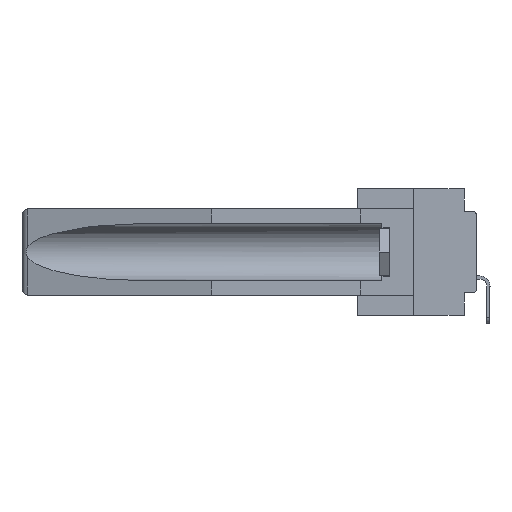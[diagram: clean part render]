
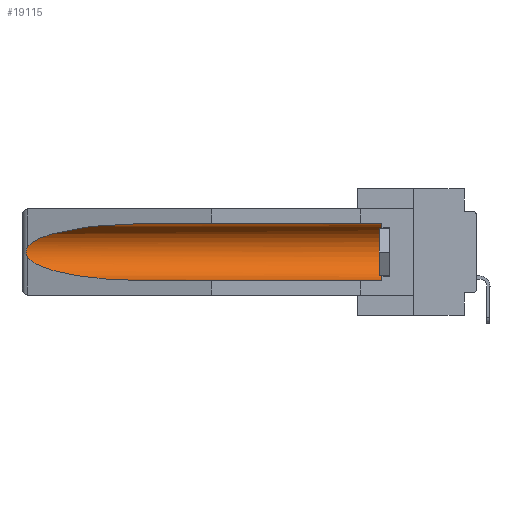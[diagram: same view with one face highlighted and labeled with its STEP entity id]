
A CAD part, left-side view. The second image highlights one B-rep face of the part: STEP entity #19115.
In plain terms, the highlighted cylindrical face has radius 2.857 mm (diameter 5.715 mm), a partial arc.
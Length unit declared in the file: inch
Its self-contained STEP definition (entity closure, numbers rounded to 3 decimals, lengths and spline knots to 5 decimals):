
#19 = ORIENTED_EDGE ( 'NONE', *, *, #5161, .T. ) ;
#198 = ORIENTED_EDGE ( 'NONE', *, *, #28148, .T. ) ;
#740 = CYLINDRICAL_SURFACE ( 'NONE', #19014, 0.1125 ) ;
#1130 = B_SPLINE_CURVE_WITH_KNOTS ( 'NONE', 3,
 ( #10382, #30782, #22417, #28241, #13743, #25695, #16826, #25834, #5448, #13874 ),
 .UNSPECIFIED., .F., .F.,
 ( 4, 2, 2, 2, 4 ),
 ( 0., 0.00029, 0.00058, 0.00087, 0.00117 ),
 .UNSPECIFIED. ) ;
#1385 = DIRECTION ( 'NONE',  ( 0., 1., 0. ) ) ;
#1723 =( BOUNDED_CURVE ( )  B_SPLINE_CURVE ( 3, ( #23127, #3036, #36189, #18755 ),
 .UNSPECIFIED., .F., .F. ) 
 B_SPLINE_CURVE_WITH_KNOTS ( ( 4, 4 ),
 ( 0.1948, 1.5708 ),
 .UNSPECIFIED. ) 
 CURVE ( )  GEOMETRIC_REPRESENTATION_ITEM ( )  RATIONAL_B_SPLINE_CURVE ( ( 1., 0.848, 0.848, 1. ) ) 
 REPRESENTATION_ITEM ( '' )  );
#3028 = ORIENTED_EDGE ( 'NONE', *, *, #11468, .T. ) ;
#3036 = CARTESIAN_POINT ( 'NONE',  ( 0.25451, 1.48313, -0.24835 ) ) ;
#4368 = CARTESIAN_POINT ( 'NONE',  ( 0.21114, 1.30732, -0.059 ) ) ;
#5161 = EDGE_CURVE ( 'NONE', #23749, #19761, #11423, .T. ) ;
#5400 = CARTESIAN_POINT ( 'NONE',  ( 0.155, 1.07973, -0.059 ) ) ;
#5448 = CARTESIAN_POINT ( 'NONE',  ( 0.26597, 1.5296, -0.19026 ) ) ;
#6351 = VERTEX_POINT ( 'NONE', #31432 ) ;
#9955 = CARTESIAN_POINT ( 'NONE',  ( 0.155, 1.07973, -0.059 ) ) ;
#10213 = CARTESIAN_POINT ( 'NONE',  ( 0.26537, 1.52718, -0.14972 ) ) ;
#10382 = CARTESIAN_POINT ( 'NONE',  ( 0.26537, 1.52718, -0.14972 ) ) ;
#11423 = CIRCLE ( 'NONE', #29286, 0.1125 ) ;
#11467 = EDGE_CURVE ( 'NONE', #19761, #15200, #25414, .T. ) ;
#11468 = EDGE_CURVE ( 'NONE', #15200, #33629, #28291, .T. ) ;
#12829 = DIRECTION ( 'NONE',  ( 0., 1., 0. ) ) ;
#13580 = EDGE_LOOP ( 'NONE', ( #3028, #198, #37270, #25937, #19, #24057 ) ) ;
#13743 = CARTESIAN_POINT ( 'NONE',  ( 0.2675, 1.53308, -0.16763 ) ) ;
#13874 = CARTESIAN_POINT ( 'NONE',  ( 0.26537, 1.52718, -0.19328 ) ) ;
#14244 = CARTESIAN_POINT ( 'NONE',  ( 0.26537, 1.52718, -0.14972 ) ) ;
#15200 = VERTEX_POINT ( 'NONE', #5400 ) ;
#15215 = EDGE_CURVE ( 'NONE', #32566, #6351, #1723, .T. ) ;
#15231 = CARTESIAN_POINT ( 'NONE',  ( 0.155, -0.30754, -0.284 ) ) ;
#15572 = DIRECTION ( 'NONE',  ( 0., 1., 0. ) ) ;
#16826 = CARTESIAN_POINT ( 'NONE',  ( 0.2673, 1.53269, -0.17917 ) ) ;
#17711 = VECTOR ( 'NONE', #12829, 39.37008 ) ;
#18595 = EDGE_CURVE ( 'NONE', #23749, #6351, #22329, .T. ) ;
#18675 = CARTESIAN_POINT ( 'NONE',  ( 0.155, 0.126, -0.1715 ) ) ;
#18755 = CARTESIAN_POINT ( 'NONE',  ( 0.155, 1.07973, -0.284 ) ) ;
#19014 = AXIS2_PLACEMENT_3D ( 'NONE', #36340, #1385, #21835 ) ;
#19115 = ADVANCED_FACE ( 'NONE', ( #36886 ), #740, .F. ) ;
#19761 = VERTEX_POINT ( 'NONE', #23726 ) ;
#21835 = DIRECTION ( 'NONE',  ( 0., 0., 1. ) ) ;
#22329 = LINE ( 'NONE', #15231, #17711 ) ;
#22417 = CARTESIAN_POINT ( 'NONE',  ( 0.26654, 1.53092, -0.15636 ) ) ;
#23127 = CARTESIAN_POINT ( 'NONE',  ( 0.26537, 1.52718, -0.19328 ) ) ;
#23726 = CARTESIAN_POINT ( 'NONE',  ( 0.155, 0.126, -0.059 ) ) ;
#23749 = VERTEX_POINT ( 'NONE', #36259 ) ;
#24057 = ORIENTED_EDGE ( 'NONE', *, *, #11467, .T. ) ;
#24253 = DIRECTION ( 'NONE',  ( 0., 0., 1. ) ) ;
#24376 = CARTESIAN_POINT ( 'NONE',  ( 0.155, -0.30754, -0.059 ) ) ;
#25414 = LINE ( 'NONE', #24376, #29894 ) ;
#25695 = CARTESIAN_POINT ( 'NONE',  ( 0.2675, 1.53308, -0.17534 ) ) ;
#25834 = CARTESIAN_POINT ( 'NONE',  ( 0.26655, 1.53094, -0.18657 ) ) ;
#25937 = ORIENTED_EDGE ( 'NONE', *, *, #18595, .F. ) ;
#28148 = EDGE_CURVE ( 'NONE', #33629, #32566, #1130, .T. ) ;
#28241 = CARTESIAN_POINT ( 'NONE',  ( 0.2673, 1.5327, -0.16383 ) ) ;
#28291 =( BOUNDED_CURVE ( )  B_SPLINE_CURVE ( 3, ( #9955, #4368, #36365, #10213 ),
 .UNSPECIFIED., .F., .F. ) 
 B_SPLINE_CURVE_WITH_KNOTS ( ( 4, 4 ),
 ( 4.71239, 6.08839 ),
 .UNSPECIFIED. ) 
 CURVE ( )  GEOMETRIC_REPRESENTATION_ITEM ( )  RATIONAL_B_SPLINE_CURVE ( ( 1., 0.848, 0.848, 1. ) ) 
 REPRESENTATION_ITEM ( '' )  );
#29239 = CARTESIAN_POINT ( 'NONE',  ( 0.26537, 1.52718, -0.19328 ) ) ;
#29286 = AXIS2_PLACEMENT_3D ( 'NONE', #18675, #35831, #24253 ) ;
#29894 = VECTOR ( 'NONE', #15572, 39.37008 ) ;
#30782 = CARTESIAN_POINT ( 'NONE',  ( 0.26597, 1.52961, -0.15275 ) ) ;
#31432 = CARTESIAN_POINT ( 'NONE',  ( 0.155, 1.07973, -0.284 ) ) ;
#32566 = VERTEX_POINT ( 'NONE', #29239 ) ;
#33629 = VERTEX_POINT ( 'NONE', #14244 ) ;
#35831 = DIRECTION ( 'NONE',  ( 0., -1., 0. ) ) ;
#36189 = CARTESIAN_POINT ( 'NONE',  ( 0.21114, 1.30732, -0.284 ) ) ;
#36259 = CARTESIAN_POINT ( 'NONE',  ( 0.155, 0.126, -0.284 ) ) ;
#36340 = CARTESIAN_POINT ( 'NONE',  ( 0.155, -0.30754, -0.1715 ) ) ;
#36365 = CARTESIAN_POINT ( 'NONE',  ( 0.25451, 1.48313, -0.09465 ) ) ;
#36886 = FACE_OUTER_BOUND ( 'NONE', #13580, .T. ) ;
#37270 = ORIENTED_EDGE ( 'NONE', *, *, #15215, .T. ) ;
